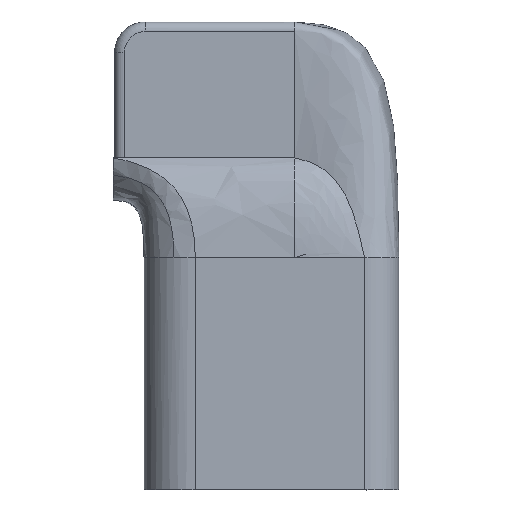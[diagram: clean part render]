
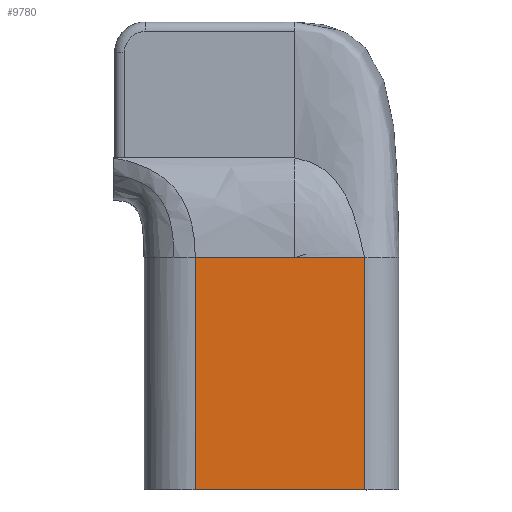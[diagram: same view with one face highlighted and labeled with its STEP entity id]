
A CAD part, left-side view. The second image highlights one B-rep face of the part: STEP entity #9780.
In plain terms, the highlighted planar face has unit normal (-1, 0, 0).
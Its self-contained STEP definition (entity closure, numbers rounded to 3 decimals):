
#299 = VECTOR ( 'NONE', #19142, 1000. ) ;
#4724 = CARTESIAN_POINT ( 'NONE',  ( -18.567, 12.147, -48.148 ) ) ;
#4798 = EDGE_LOOP ( 'NONE', ( #7846, #11511, #16141, #7012, #21171 ) ) ;
#4876 = CARTESIAN_POINT ( 'NONE',  ( -18.567, -10.64, -48.148 ) ) ;
#5006 = DIRECTION ( 'NONE',  ( 0., -1., 0. ) ) ;
#5675 = CARTESIAN_POINT ( 'NONE',  ( -18.567, -45.775, 0. ) ) ;
#6198 = LINE ( 'NONE', #4724, #6779 ) ;
#6464 = LINE ( 'NONE', #11675, #299 ) ;
#6520 = VERTEX_POINT ( 'NONE', #21312 ) ;
#6627 = CARTESIAN_POINT ( 'NONE',  ( -18.567, -10.64, 162.309 ) ) ;
#6779 = VECTOR ( 'NONE', #15975, 1000. ) ;
#7012 = ORIENTED_EDGE ( 'NONE', *, *, #19402, .T. ) ;
#7164 = CARTESIAN_POINT ( 'NONE',  ( -18.567, -40.912, 0. ) ) ;
#7458 = CARTESIAN_POINT ( 'NONE',  ( -18.567, -45.775, -48.148 ) ) ;
#7846 = ORIENTED_EDGE ( 'NONE', *, *, #18969, .T. ) ;
#8171 = VERTEX_POINT ( 'NONE', #16995 ) ;
#8530 = DIRECTION ( 'NONE',  ( 0., 0., -1. ) ) ;
#8534 = VECTOR ( 'NONE', #8530, 1000. ) ;
#8621 = CARTESIAN_POINT ( 'NONE',  ( -18.567, -45.775, 162.309 ) ) ;
#9119 = AXIS2_PLACEMENT_3D ( 'NONE', #8621, #21740, #10512 ) ;
#9780 = ADVANCED_FACE ( 'NONE', ( #16570 ), #19872, .T. ) ;
#10512 = DIRECTION ( 'NONE',  ( 0., 0., 1. ) ) ;
#10958 = CARTESIAN_POINT ( 'NONE',  ( -18.567, -36.049, 0. ) ) ;
#11372 = LINE ( 'NONE', #16247, #21352 ) ;
#11511 = ORIENTED_EDGE ( 'NONE', *, *, #17348, .F. ) ;
#11575 = VERTEX_POINT ( 'NONE', #4876 ) ;
#11675 = CARTESIAN_POINT ( 'NONE',  ( -18.567, -45.775, 162.309 ) ) ;
#12081 = VERTEX_POINT ( 'NONE', #5675 ) ;
#15975 = DIRECTION ( 'NONE',  ( 0., 1., 0. ) ) ;
#16141 = ORIENTED_EDGE ( 'NONE', *, *, #18751, .T. ) ;
#16247 = CARTESIAN_POINT ( 'NONE',  ( -18.567, 16.066, 0. ) ) ;
#16570 = FACE_OUTER_BOUND ( 'NONE', #4798, .T. ) ;
#16995 = CARTESIAN_POINT ( 'NONE',  ( -18.567, -31.186, 0. ) ) ;
#17348 = EDGE_CURVE ( 'NONE', #20551, #11575, #6198, .T. ) ;
#18519 = LINE ( 'NONE', #6627, #8534 ) ;
#18751 = EDGE_CURVE ( 'NONE', #20551, #12081, #6464, .T. ) ;
#18969 = EDGE_CURVE ( 'NONE', #6520, #11575, #18519, .T. ) ;
#19142 = DIRECTION ( 'NONE',  ( 0., 0., 1. ) ) ;
#19402 = EDGE_CURVE ( 'NONE', #12081, #8171, #21818, .T. ) ;
#19872 = PLANE ( 'NONE',  #9119 ) ;
#20313 = CARTESIAN_POINT ( 'NONE',  ( -18.567, -45.775, 0. ) ) ;
#20551 = VERTEX_POINT ( 'NONE', #7458 ) ;
#21171 = ORIENTED_EDGE ( 'NONE', *, *, #22705, .F. ) ;
#21312 = CARTESIAN_POINT ( 'NONE',  ( -18.567, -10.64, 0. ) ) ;
#21352 = VECTOR ( 'NONE', #5006, 1000. ) ;
#21740 = DIRECTION ( 'NONE',  ( -1., 0., 0. ) ) ;
#21818 = B_SPLINE_CURVE_WITH_KNOTS ( 'NONE', 3,
 ( #20313, #7164, #10958, #24086 ),
 .UNSPECIFIED., .F., .F.,
 ( 4, 4 ),
 ( 0., 1. ),
 .UNSPECIFIED. ) ;
#22705 = EDGE_CURVE ( 'NONE', #6520, #8171, #11372, .T. ) ;
#24086 = CARTESIAN_POINT ( 'NONE',  ( -18.567, -31.186, 0. ) ) ;
